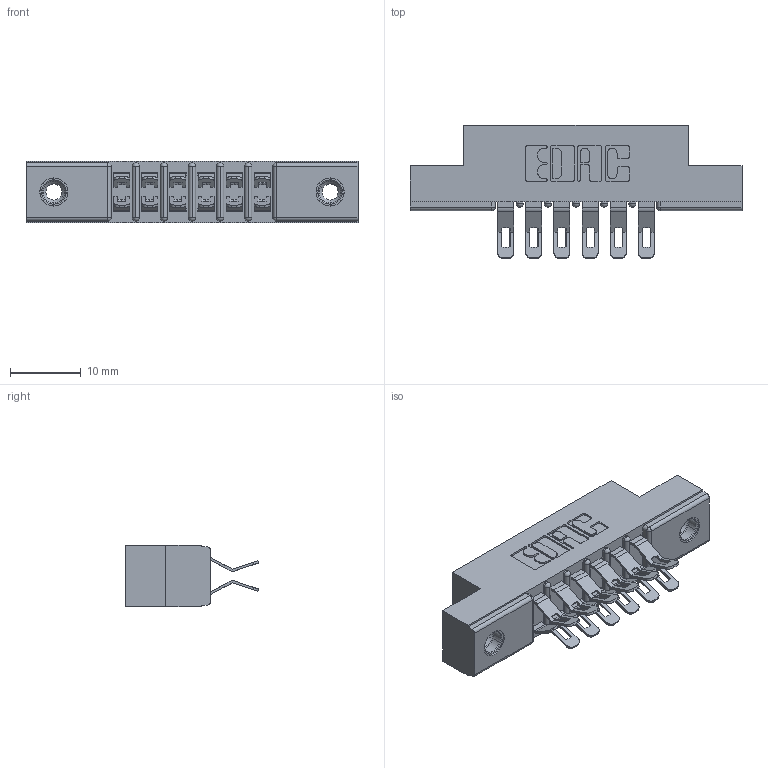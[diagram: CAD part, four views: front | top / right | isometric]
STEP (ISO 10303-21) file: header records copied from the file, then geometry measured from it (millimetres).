
FILE_DESCRIPTION (( 'STEP AP203' ), '1' );
FILE_NAME ('357-012-455-208.STEP', '2020-10-02T16:35:57', ( '' ), ( '' ), 'SwSTEP 2.0', 'SolidWorks 2020', '' );
FILE_SCHEMA (( 'CONFIG_CONTROL_DESIGN' ));
Length unit declared in the file: inch
Products named in the file (4): 307 Part_.156 Dia Mounting Holes; 307-290-001_555; 357-012-455-208; 345-250-001_345-250-003-102
Assembly tree (15 placements, depth 2):
  357-012-455-208
    307 Part_.156 Dia Mounting Holes
    307-290-001_555  x12
    345-250-001_345-250-003-102  x2
Bounding box: 46.79 x 18.75 x 8.71 mm (x, y, z)
Volume: 3091.4 mm3; surface area: 4844.9 mm2
Topology: 15 solids, 15 shells, 917 faces, 2631 edges, 1710 vertices
Faces by surface type: plane 510, cylinder 377, sphere 14, cone 12, torus 4
Entity records: 11496 total; most frequent: CARTESIAN_POINT 1881, DIRECTION 1874, ORIENTED_EDGE 1856, EDGE_CURVE 928, VECTOR 684, LINE 684, VERTEX_POINT 602, AXIS2_PLACEMENT_3D 595
